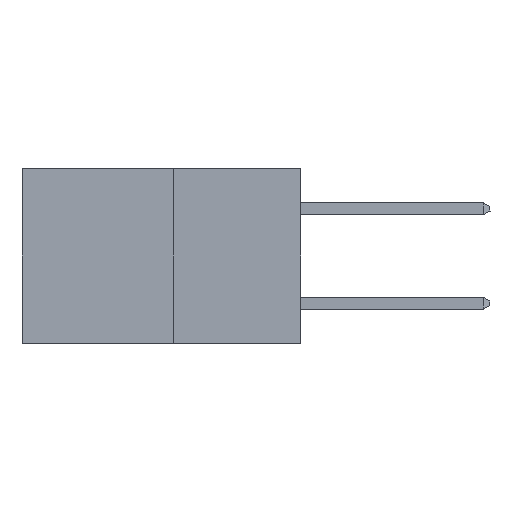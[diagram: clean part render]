
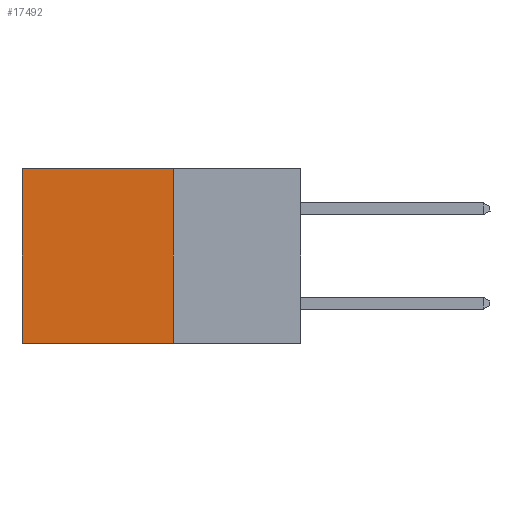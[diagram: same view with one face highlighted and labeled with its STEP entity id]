
A CAD part, left-side view. The second image highlights one B-rep face of the part: STEP entity #17492.
In plain terms, the highlighted planar face has unit normal (-1, 0, 0).
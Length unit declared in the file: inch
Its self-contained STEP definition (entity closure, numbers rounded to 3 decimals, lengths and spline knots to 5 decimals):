
#311 = DIRECTION ( 'NONE',  ( 0., 1., 0. ) ) ;
#598 = LINE ( 'NONE', #6929, #10882 ) ;
#943 = CARTESIAN_POINT ( 'NONE',  ( 0.277, 0.27, 0. ) ) ;
#1346 = FACE_OUTER_BOUND ( 'NONE', #12644, .T. ) ;
#2578 = EDGE_CURVE ( 'NONE', #4838, #13002, #4791, .T. ) ;
#2647 = CARTESIAN_POINT ( 'NONE',  ( 0.277, 0.27, 0. ) ) ;
#2879 = VERTEX_POINT ( 'NONE', #17303 ) ;
#3827 = EDGE_CURVE ( 'NONE', #4838, #9808, #9774, .T. ) ;
#4791 = LINE ( 'NONE', #17247, #11286 ) ;
#4838 = VERTEX_POINT ( 'NONE', #2647 ) ;
#6929 = CARTESIAN_POINT ( 'NONE',  ( 0.277, 0.27, -0.37 ) ) ;
#7705 = LINE ( 'NONE', #9207, #14509 ) ;
#8230 = CARTESIAN_POINT ( 'NONE',  ( 0.277, 0.27, -0.37 ) ) ;
#8561 = EDGE_CURVE ( 'NONE', #13002, #2879, #598, .T. ) ;
#8747 = DIRECTION ( 'NONE',  ( 0., 0., -1. ) ) ;
#9207 = CARTESIAN_POINT ( 'NONE',  ( 0.277, 0.59, -0.37 ) ) ;
#9255 = ORIENTED_EDGE ( 'NONE', *, *, #13656, .T. ) ;
#9774 = LINE ( 'NONE', #943, #12963 ) ;
#9808 = VERTEX_POINT ( 'NONE', #12682 ) ;
#10882 = VECTOR ( 'NONE', #311, 39.37008 ) ;
#11196 = ORIENTED_EDGE ( 'NONE', *, *, #8561, .F. ) ;
#11286 = VECTOR ( 'NONE', #15796, 39.37008 ) ;
#11541 = DIRECTION ( 'NONE',  ( 0., 0., -1. ) ) ;
#11561 = DIRECTION ( 'NONE',  ( 1., 0., 0. ) ) ;
#11617 = PLANE ( 'NONE',  #13740 ) ;
#11635 = DIRECTION ( 'NONE',  ( 0., 1., 0. ) ) ;
#11931 = CARTESIAN_POINT ( 'NONE',  ( 0.277, 0.27, -0.37 ) ) ;
#12644 = EDGE_LOOP ( 'NONE', ( #9255, #11196, #14377, #17330 ) ) ;
#12682 = CARTESIAN_POINT ( 'NONE',  ( 0.277, 0.59, 0. ) ) ;
#12963 = VECTOR ( 'NONE', #11635, 39.37008 ) ;
#13002 = VERTEX_POINT ( 'NONE', #8230 ) ;
#13656 = EDGE_CURVE ( 'NONE', #9808, #2879, #7705, .T. ) ;
#13740 = AXIS2_PLACEMENT_3D ( 'NONE', #11931, #11561, #11541 ) ;
#14377 = ORIENTED_EDGE ( 'NONE', *, *, #2578, .F. ) ;
#14509 = VECTOR ( 'NONE', #8747, 39.37008 ) ;
#15796 = DIRECTION ( 'NONE',  ( 0., 0., -1. ) ) ;
#17247 = CARTESIAN_POINT ( 'NONE',  ( 0.277, 0.27, -0.37 ) ) ;
#17303 = CARTESIAN_POINT ( 'NONE',  ( 0.277, 0.59, -0.37 ) ) ;
#17330 = ORIENTED_EDGE ( 'NONE', *, *, #3827, .T. ) ;
#17492 = ADVANCED_FACE ( 'NONE', ( #1346 ), #11617, .F. ) ;
